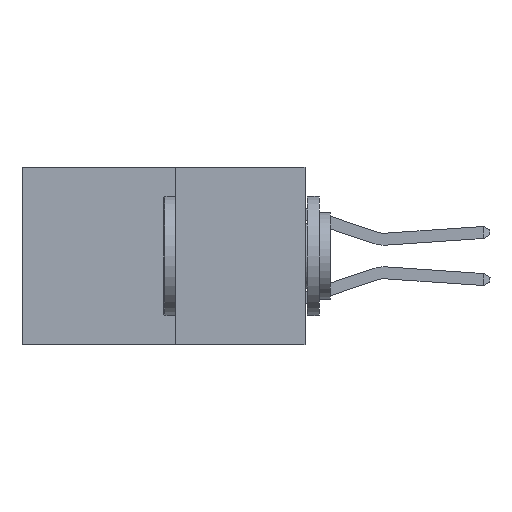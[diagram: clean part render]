
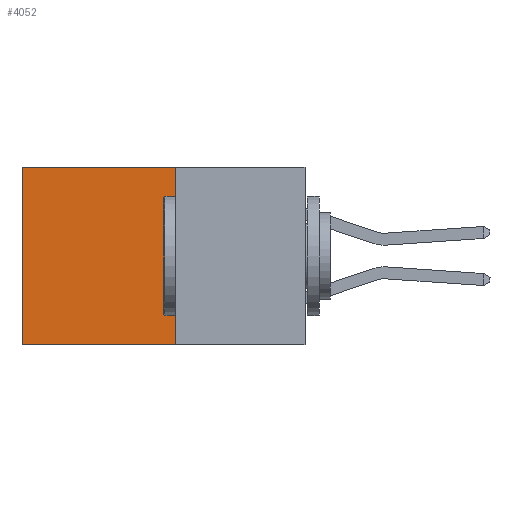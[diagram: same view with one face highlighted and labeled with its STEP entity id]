
A CAD part, left-side view. The second image highlights one B-rep face of the part: STEP entity #4052.
In plain terms, the highlighted planar face has unit normal (-1, 0, 0).
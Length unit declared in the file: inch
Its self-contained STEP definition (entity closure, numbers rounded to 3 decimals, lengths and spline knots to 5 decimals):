
#150 = VERTEX_POINT ( 'NONE', #22482 ) ;
#446 = LINE ( 'NONE', #1692, #20156 ) ;
#1175 = LINE ( 'NONE', #13549, #8104 ) ;
#1692 = CARTESIAN_POINT ( 'NONE',  ( 0.277, 0.59, -0.37 ) ) ;
#2734 = PLANE ( 'NONE',  #19338 ) ;
#3434 = VECTOR ( 'NONE', #22267, 39.37008 ) ;
#3963 = CARTESIAN_POINT ( 'NONE',  ( 0.277, 0.27, 0. ) ) ;
#4052 = ADVANCED_FACE ( 'NONE', ( #14400 ), #2734, .F. ) ;
#5789 = EDGE_CURVE ( 'NONE', #21130, #150, #1175, .T. ) ;
#5873 = DIRECTION ( 'NONE',  ( 0., 1., 0. ) ) ;
#6621 = DIRECTION ( 'NONE',  ( 0., 0., -1. ) ) ;
#8104 = VECTOR ( 'NONE', #5873, 39.37008 ) ;
#8567 = LINE ( 'NONE', #8929, #3434 ) ;
#8734 = VECTOR ( 'NONE', #19449, 39.37008 ) ;
#8929 = CARTESIAN_POINT ( 'NONE',  ( 0.277, 0.27, -0.37 ) ) ;
#9094 = ORIENTED_EDGE ( 'NONE', *, *, #14397, .F. ) ;
#10964 = EDGE_CURVE ( 'NONE', #21130, #17135, #24355, .T. ) ;
#13445 = ORIENTED_EDGE ( 'NONE', *, *, #5789, .T. ) ;
#13549 = CARTESIAN_POINT ( 'NONE',  ( 0.277, 0.27, 0. ) ) ;
#14397 = EDGE_CURVE ( 'NONE', #17135, #18188, #8567, .T. ) ;
#14400 = FACE_OUTER_BOUND ( 'NONE', #17109, .T. ) ;
#14537 = EDGE_CURVE ( 'NONE', #150, #18188, #446, .T. ) ;
#16110 = CARTESIAN_POINT ( 'NONE',  ( 0.277, 0.27, -0.37 ) ) ;
#16995 = DIRECTION ( 'NONE',  ( 0., 0., -1. ) ) ;
#17033 = CARTESIAN_POINT ( 'NONE',  ( 0.277, 0.59, -0.37 ) ) ;
#17109 = EDGE_LOOP ( 'NONE', ( #23912, #9094, #22774, #13445 ) ) ;
#17135 = VERTEX_POINT ( 'NONE', #23616 ) ;
#17540 = CARTESIAN_POINT ( 'NONE',  ( 0.277, 0.27, -0.37 ) ) ;
#18009 = DIRECTION ( 'NONE',  ( 1., 0., 0. ) ) ;
#18188 = VERTEX_POINT ( 'NONE', #17033 ) ;
#19338 = AXIS2_PLACEMENT_3D ( 'NONE', #16110, #18009, #6621 ) ;
#19449 = DIRECTION ( 'NONE',  ( 0., 0., -1. ) ) ;
#20156 = VECTOR ( 'NONE', #16995, 39.37008 ) ;
#21130 = VERTEX_POINT ( 'NONE', #3963 ) ;
#22267 = DIRECTION ( 'NONE',  ( 0., 1., 0. ) ) ;
#22482 = CARTESIAN_POINT ( 'NONE',  ( 0.277, 0.59, 0. ) ) ;
#22774 = ORIENTED_EDGE ( 'NONE', *, *, #10964, .F. ) ;
#23616 = CARTESIAN_POINT ( 'NONE',  ( 0.277, 0.27, -0.37 ) ) ;
#23912 = ORIENTED_EDGE ( 'NONE', *, *, #14537, .T. ) ;
#24355 = LINE ( 'NONE', #17540, #8734 ) ;
